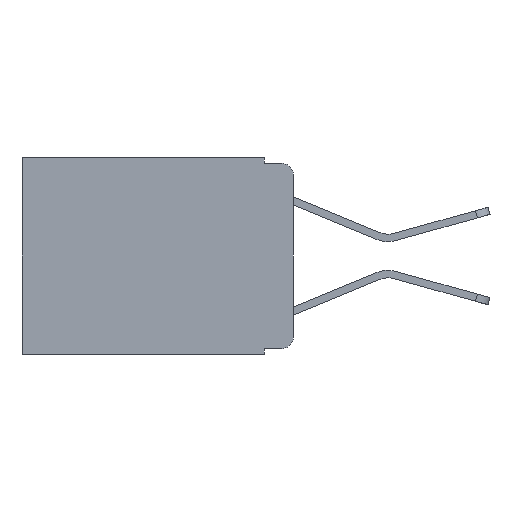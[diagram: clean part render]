
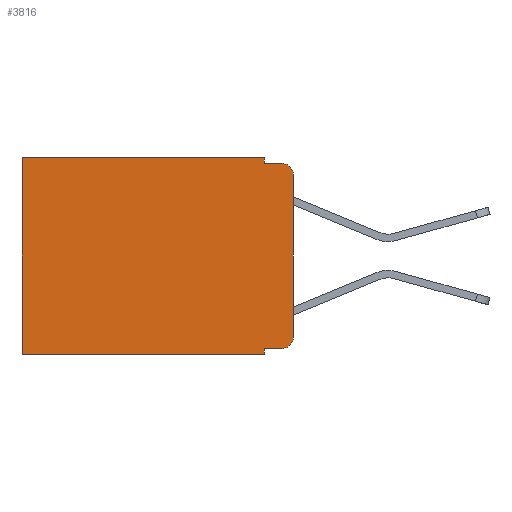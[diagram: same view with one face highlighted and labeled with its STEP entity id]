
A CAD part, left-side view. The second image highlights one B-rep face of the part: STEP entity #3816.
In plain terms, the highlighted planar face has unit normal (-1, 0, 0).
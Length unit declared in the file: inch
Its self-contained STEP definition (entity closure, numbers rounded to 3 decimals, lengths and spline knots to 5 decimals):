
#10 = EDGE_CURVE ( 'NONE', #12107, #11976, #1262, .T. ) ;
#347 = EDGE_CURVE ( 'NONE', #5121, #855, #8970, .T. ) ;
#388 = DIRECTION ( 'NONE',  ( 0., 0., -1. ) ) ;
#543 = ORIENTED_EDGE ( 'NONE', *, *, #11491, .T. ) ;
#847 = CARTESIAN_POINT ( 'NONE',  ( 0.298, 0., -0.343 ) ) ;
#855 = VERTEX_POINT ( 'NONE', #2195 ) ;
#929 = CARTESIAN_POINT ( 'NONE',  ( 0.298, 0., -0.03 ) ) ;
#1101 = DIRECTION ( 'NONE',  ( -1., 0., 0. ) ) ;
#1175 = VECTOR ( 'NONE', #6312, 39.37008 ) ;
#1262 = CIRCLE ( 'NONE', #10858, 0.02 ) ;
#1322 = DIRECTION ( 'NONE',  ( -1., 0., 0. ) ) ;
#1424 = VECTOR ( 'NONE', #8968, 39.37008 ) ;
#1588 = CARTESIAN_POINT ( 'NONE',  ( 0.298, 0., 0. ) ) ;
#1654 = ORIENTED_EDGE ( 'NONE', *, *, #5473, .T. ) ;
#1765 = ORIENTED_EDGE ( 'NONE', *, *, #10268, .F. ) ;
#1803 = CARTESIAN_POINT ( 'NONE',  ( 0.298, 0.473, 0. ) ) ;
#1866 = VECTOR ( 'NONE', #11545, 39.37008 ) ;
#2195 = CARTESIAN_POINT ( 'NONE',  ( 0.298, 0.02, -0.01 ) ) ;
#2212 = DIRECTION ( 'NONE',  ( 1., 0., 0. ) ) ;
#2267 = CARTESIAN_POINT ( 'NONE',  ( 0.298, 0., -0.313 ) ) ;
#2391 = CARTESIAN_POINT ( 'NONE',  ( 0.298, 0.02, -0.333 ) ) ;
#2488 = CARTESIAN_POINT ( 'NONE',  ( 0.298, 0., 0. ) ) ;
#2768 = CARTESIAN_POINT ( 'NONE',  ( 0.298, 0.051, -0.01 ) ) ;
#2779 = ORIENTED_EDGE ( 'NONE', *, *, #3619, .F. ) ;
#2915 = EDGE_CURVE ( 'NONE', #3858, #6491, #5235, .T. ) ;
#3505 = VECTOR ( 'NONE', #10261, 39.37008 ) ;
#3520 = ORIENTED_EDGE ( 'NONE', *, *, #8674, .T. ) ;
#3619 = EDGE_CURVE ( 'NONE', #5009, #5121, #7130, .T. ) ;
#3661 = CARTESIAN_POINT ( 'NONE',  ( 0.298, 0.051, 0. ) ) ;
#3816 = ADVANCED_FACE ( 'NONE', ( #6981 ), #9120, .F. ) ;
#3858 = VERTEX_POINT ( 'NONE', #12320 ) ;
#4167 = CARTESIAN_POINT ( 'NONE',  ( 0.298, 0.02, -0.313 ) ) ;
#4628 = LINE ( 'NONE', #847, #11634 ) ;
#4761 = EDGE_CURVE ( 'NONE', #5304, #11976, #6160, .T. ) ;
#4887 = DIRECTION ( 'NONE',  ( 0., 0., -1. ) ) ;
#5009 = VERTEX_POINT ( 'NONE', #3661 ) ;
#5014 = ORIENTED_EDGE ( 'NONE', *, *, #10, .T. ) ;
#5121 = VERTEX_POINT ( 'NONE', #2768 ) ;
#5235 = LINE ( 'NONE', #10964, #9638 ) ;
#5304 = VERTEX_POINT ( 'NONE', #929 ) ;
#5466 = VECTOR ( 'NONE', #4887, 39.37008 ) ;
#5473 = EDGE_CURVE ( 'NONE', #5304, #855, #7779, .T. ) ;
#5727 = VERTEX_POINT ( 'NONE', #7041 ) ;
#5797 = DIRECTION ( 'NONE',  ( 0., 0., -1. ) ) ;
#6160 = LINE ( 'NONE', #7107, #1424 ) ;
#6312 = DIRECTION ( 'NONE',  ( 0., -1., 0. ) ) ;
#6430 = ORIENTED_EDGE ( 'NONE', *, *, #2915, .F. ) ;
#6491 = VERTEX_POINT ( 'NONE', #10151 ) ;
#6537 = LINE ( 'NONE', #10891, #1175 ) ;
#6618 = CARTESIAN_POINT ( 'NONE',  ( 0.298, 0.051, 0. ) ) ;
#6966 = VERTEX_POINT ( 'NONE', #8910 ) ;
#6981 = FACE_OUTER_BOUND ( 'NONE', #10324, .T. ) ;
#7003 = VECTOR ( 'NONE', #11025, 39.37008 ) ;
#7041 = CARTESIAN_POINT ( 'NONE',  ( 0.298, 0.473, -0.343 ) ) ;
#7107 = CARTESIAN_POINT ( 'NONE',  ( 0.298, 0., 0. ) ) ;
#7130 = LINE ( 'NONE', #6618, #1866 ) ;
#7286 = CARTESIAN_POINT ( 'NONE',  ( 0.298, 0.02, -0.03 ) ) ;
#7288 = LINE ( 'NONE', #2488, #7003 ) ;
#7779 = CIRCLE ( 'NONE', #9981, 0.02 ) ;
#7796 = DIRECTION ( 'NONE',  ( 0., 1., 0. ) ) ;
#8255 = DIRECTION ( 'NONE',  ( 0., 0., -1. ) ) ;
#8299 = LINE ( 'NONE', #1803, #5466 ) ;
#8432 = EDGE_CURVE ( 'NONE', #3858, #12107, #6537, .T. ) ;
#8624 = AXIS2_PLACEMENT_3D ( 'NONE', #1588, #2212, #12011 ) ;
#8674 = EDGE_CURVE ( 'NONE', #6966, #5727, #8299, .T. ) ;
#8910 = CARTESIAN_POINT ( 'NONE',  ( 0.298, 0.473, 0. ) ) ;
#8968 = DIRECTION ( 'NONE',  ( 0., 0., -1. ) ) ;
#8970 = LINE ( 'NONE', #10279, #3505 ) ;
#9120 = PLANE ( 'NONE',  #8624 ) ;
#9418 = ORIENTED_EDGE ( 'NONE', *, *, #347, .F. ) ;
#9638 = VECTOR ( 'NONE', #5797, 39.37008 ) ;
#9699 = ORIENTED_EDGE ( 'NONE', *, *, #4761, .F. ) ;
#9981 = AXIS2_PLACEMENT_3D ( 'NONE', #7286, #1322, #8255 ) ;
#10151 = CARTESIAN_POINT ( 'NONE',  ( 0.298, 0.051, -0.343 ) ) ;
#10261 = DIRECTION ( 'NONE',  ( 0., -1., 0. ) ) ;
#10268 = EDGE_CURVE ( 'NONE', #6491, #5727, #4628, .T. ) ;
#10279 = CARTESIAN_POINT ( 'NONE',  ( 0.298, 0.051, -0.01 ) ) ;
#10324 = EDGE_LOOP ( 'NONE', ( #9699, #1654, #9418, #2779, #543, #3520, #1765, #6430, #10531, #5014 ) ) ;
#10531 = ORIENTED_EDGE ( 'NONE', *, *, #8432, .T. ) ;
#10858 = AXIS2_PLACEMENT_3D ( 'NONE', #4167, #1101, #388 ) ;
#10891 = CARTESIAN_POINT ( 'NONE',  ( 0.298, 0.051, -0.333 ) ) ;
#10964 = CARTESIAN_POINT ( 'NONE',  ( 0.298, 0.051, 0. ) ) ;
#11025 = DIRECTION ( 'NONE',  ( 0., 1., 0. ) ) ;
#11491 = EDGE_CURVE ( 'NONE', #5009, #6966, #7288, .T. ) ;
#11545 = DIRECTION ( 'NONE',  ( 0., 0., -1. ) ) ;
#11634 = VECTOR ( 'NONE', #7796, 39.37008 ) ;
#11976 = VERTEX_POINT ( 'NONE', #2267 ) ;
#12011 = DIRECTION ( 'NONE',  ( 0., 0., -1. ) ) ;
#12107 = VERTEX_POINT ( 'NONE', #2391 ) ;
#12320 = CARTESIAN_POINT ( 'NONE',  ( 0.298, 0.051, -0.333 ) ) ;
